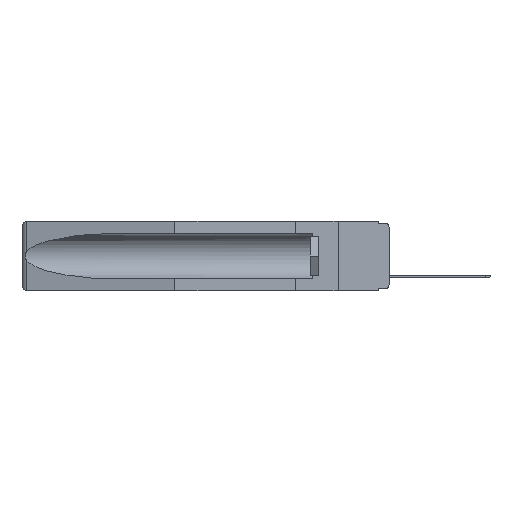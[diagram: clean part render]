
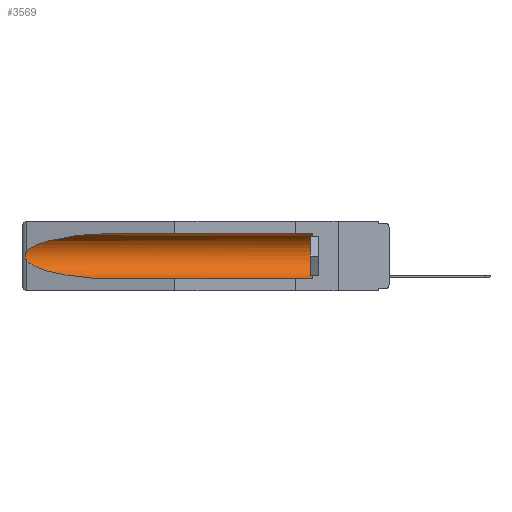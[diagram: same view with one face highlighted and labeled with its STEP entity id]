
A CAD part, left-side view. The second image highlights one B-rep face of the part: STEP entity #3569.
In plain terms, the highlighted cylindrical face has radius 2.857 mm (diameter 5.715 mm), a partial arc.
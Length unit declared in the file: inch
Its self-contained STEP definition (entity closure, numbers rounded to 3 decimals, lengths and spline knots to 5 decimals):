
#88 = AXIS2_PLACEMENT_3D ( 'NONE', #10822, #1616, #197 ) ;
#93 = CARTESIAN_POINT ( 'NONE',  ( 0.26537, 1.52718, -0.14972 ) ) ;
#121 =( BOUNDED_CURVE ( )  B_SPLINE_CURVE ( 3, ( #11089, #5637, #602, #18111 ),
 .UNSPECIFIED., .F., .T. ) 
 B_SPLINE_CURVE_WITH_KNOTS ( ( 4, 4 ),
 ( 0.1948, 1.5708 ),
 .UNSPECIFIED. ) 
 CURVE ( )  GEOMETRIC_REPRESENTATION_ITEM ( )  RATIONAL_B_SPLINE_CURVE ( ( 1., 0.848, 0.848, 1. ) ) 
 REPRESENTATION_ITEM ( '' )  );
#197 = DIRECTION ( 'NONE',  ( 0., 0., 1. ) ) ;
#432 = CARTESIAN_POINT ( 'NONE',  ( 0.26655, 1.53094, -0.18657 ) ) ;
#602 = CARTESIAN_POINT ( 'NONE',  ( 0.21114, 1.30732, -0.284 ) ) ;
#673 = VERTEX_POINT ( 'NONE', #20935 ) ;
#872 = DIRECTION ( 'NONE',  ( 0., 1., 0. ) ) ;
#1616 = DIRECTION ( 'NONE',  ( 0., 1., 0. ) ) ;
#1844 = CARTESIAN_POINT ( 'NONE',  ( 0.26654, 1.53092, -0.15636 ) ) ;
#3087 = LINE ( 'NONE', #16733, #8057 ) ;
#3249 = CYLINDRICAL_SURFACE ( 'NONE', #88, 0.1125 ) ;
#3569 = ADVANCED_FACE ( 'NONE', ( #8628 ), #3249, .F. ) ;
#4260 = EDGE_CURVE ( 'NONE', #10483, #673, #3087, .T. ) ;
#4326 = LINE ( 'NONE', #6454, #20472 ) ;
#4409 = EDGE_CURVE ( 'NONE', #10483, #18837, #21376, .T. ) ;
#5058 = CARTESIAN_POINT ( 'NONE',  ( 0.155, 0.126, -0.1715 ) ) ;
#5637 = CARTESIAN_POINT ( 'NONE',  ( 0.25451, 1.48313, -0.24835 ) ) ;
#6183 = CARTESIAN_POINT ( 'NONE',  ( 0.25451, 1.48313, -0.09465 ) ) ;
#6454 = CARTESIAN_POINT ( 'NONE',  ( 0.155, -0.30754, -0.059 ) ) ;
#6559 = ORIENTED_EDGE ( 'NONE', *, *, #16810, .T. ) ;
#7457 = CARTESIAN_POINT ( 'NONE',  ( 0.155, 0.126, -0.059 ) ) ;
#7961 = DIRECTION ( 'NONE',  ( 0., 1., 0. ) ) ;
#8057 = VECTOR ( 'NONE', #872, 39.37008 ) ;
#8455 = VERTEX_POINT ( 'NONE', #22101 ) ;
#8628 = FACE_OUTER_BOUND ( 'NONE', #14721, .T. ) ;
#9753 = CARTESIAN_POINT ( 'NONE',  ( 0.155, 1.07973, -0.059 ) ) ;
#10483 = VERTEX_POINT ( 'NONE', #21795 ) ;
#10822 = CARTESIAN_POINT ( 'NONE',  ( 0.155, -0.30754, -0.1715 ) ) ;
#10930 = CARTESIAN_POINT ( 'NONE',  ( 0.2673, 1.53269, -0.17917 ) ) ;
#11089 = CARTESIAN_POINT ( 'NONE',  ( 0.26537, 1.52718, -0.19328 ) ) ;
#11295 = AXIS2_PLACEMENT_3D ( 'NONE', #5058, #22775, #22996 ) ;
#12202 = EDGE_CURVE ( 'NONE', #8455, #19579, #16631, .T. ) ;
#12508 = ORIENTED_EDGE ( 'NONE', *, *, #13311, .T. ) ;
#12674 = CARTESIAN_POINT ( 'NONE',  ( 0.26537, 1.52718, -0.19328 ) ) ;
#12785 = CARTESIAN_POINT ( 'NONE',  ( 0.26597, 1.52961, -0.15275 ) ) ;
#13311 = EDGE_CURVE ( 'NONE', #14169, #8455, #22184, .T. ) ;
#14060 = ORIENTED_EDGE ( 'NONE', *, *, #4409, .T. ) ;
#14169 = VERTEX_POINT ( 'NONE', #9753 ) ;
#14721 = EDGE_LOOP ( 'NONE', ( #12508, #15247, #18708, #18868, #14060, #6559 ) ) ;
#15247 = ORIENTED_EDGE ( 'NONE', *, *, #12202, .T. ) ;
#16420 = CARTESIAN_POINT ( 'NONE',  ( 0.2675, 1.53308, -0.17534 ) ) ;
#16631 = B_SPLINE_CURVE_WITH_KNOTS ( 'NONE', 3,
 ( #93, #12785, #1844, #19585, #19921, #16420, #10930, #432, #18062, #12674 ),
 .UNSPECIFIED., .F., .F.,
 ( 4, 2, 2, 2, 4 ),
 ( 0., 0.00029, 0.00058, 0.00087, 0.00117 ),
 .UNSPECIFIED. ) ;
#16733 = CARTESIAN_POINT ( 'NONE',  ( 0.155, -0.30754, -0.284 ) ) ;
#16810 = EDGE_CURVE ( 'NONE', #18837, #14169, #4326, .T. ) ;
#18062 = CARTESIAN_POINT ( 'NONE',  ( 0.26597, 1.5296, -0.19026 ) ) ;
#18111 = CARTESIAN_POINT ( 'NONE',  ( 0.155, 1.07973, -0.284 ) ) ;
#18708 = ORIENTED_EDGE ( 'NONE', *, *, #21242, .T. ) ;
#18837 = VERTEX_POINT ( 'NONE', #7457 ) ;
#18868 = ORIENTED_EDGE ( 'NONE', *, *, #4260, .F. ) ;
#19579 = VERTEX_POINT ( 'NONE', #19780 ) ;
#19585 = CARTESIAN_POINT ( 'NONE',  ( 0.2673, 1.5327, -0.16383 ) ) ;
#19780 = CARTESIAN_POINT ( 'NONE',  ( 0.26537, 1.52718, -0.19328 ) ) ;
#19921 = CARTESIAN_POINT ( 'NONE',  ( 0.2675, 1.53308, -0.16763 ) ) ;
#20472 = VECTOR ( 'NONE', #7961, 39.37008 ) ;
#20520 = CARTESIAN_POINT ( 'NONE',  ( 0.21114, 1.30732, -0.059 ) ) ;
#20633 = CARTESIAN_POINT ( 'NONE',  ( 0.155, 1.07973, -0.059 ) ) ;
#20935 = CARTESIAN_POINT ( 'NONE',  ( 0.155, 1.07973, -0.284 ) ) ;
#21242 = EDGE_CURVE ( 'NONE', #19579, #673, #121, .T. ) ;
#21376 = CIRCLE ( 'NONE', #11295, 0.1125 ) ;
#21795 = CARTESIAN_POINT ( 'NONE',  ( 0.155, 0.126, -0.284 ) ) ;
#22101 = CARTESIAN_POINT ( 'NONE',  ( 0.26537, 1.52718, -0.14972 ) ) ;
#22184 =( BOUNDED_CURVE ( )  B_SPLINE_CURVE ( 3, ( #20633, #20520, #6183, #22490 ),
 .UNSPECIFIED., .F., .T. ) 
 B_SPLINE_CURVE_WITH_KNOTS ( ( 4, 4 ),
 ( 4.71239, 6.08839 ),
 .UNSPECIFIED. ) 
 CURVE ( )  GEOMETRIC_REPRESENTATION_ITEM ( )  RATIONAL_B_SPLINE_CURVE ( ( 1., 0.848, 0.848, 1. ) ) 
 REPRESENTATION_ITEM ( '' )  );
#22490 = CARTESIAN_POINT ( 'NONE',  ( 0.26537, 1.52718, -0.14972 ) ) ;
#22775 = DIRECTION ( 'NONE',  ( 0., -1., 0. ) ) ;
#22996 = DIRECTION ( 'NONE',  ( 0., 0., 1. ) ) ;
